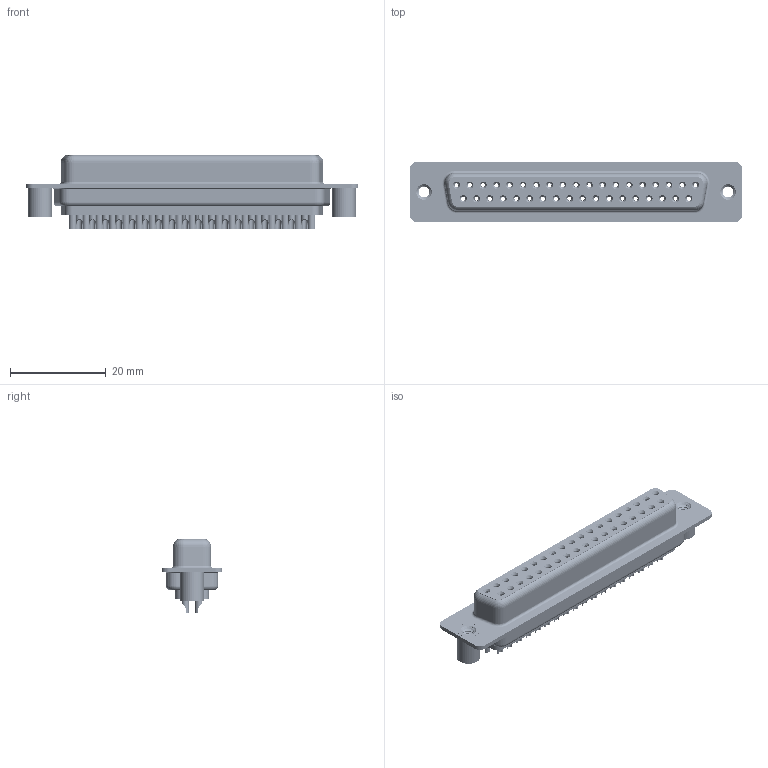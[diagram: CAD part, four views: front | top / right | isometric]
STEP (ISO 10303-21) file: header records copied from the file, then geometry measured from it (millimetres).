
FILE_DESCRIPTION (( 'STEP AP203' ), '1' );
FILE_NAME ('628-037-322-249.STEP', '2020-07-14T19:12:02', ( '' ), ( '' ), 'SwSTEP 2.0', 'SolidWorks 2020', '' );
FILE_SCHEMA (( 'CONFIG_CONTROL_DESIGN' ));
Length unit declared in the file: millimetre
Products named in the file (7): 628 Contact Row 2_22L; 628 Contact Row 1_22L; 628 4-40 Threaded Standoff BS; 628 Shell Front_37 Contacts; 628-037-322-249; 628 Shell Rear_37 Contacts; 628 Housing_37 LP
Assembly tree (42 placements, depth 2):
  628-037-322-249
    628 Housing_37 LP
    628 Shell Front_37 Contacts
    628 Shell Rear_37 Contacts
    628 Contact Row 1_22L  x19
    628 Contact Row 2_22L  x18
    628 4-40 Threaded Standoff BS  x2
Bounding box: 69.3 x 12.6 x 15.35 mm (x, y, z)
Volume: 5487.7 mm3; surface area: 13204.8 mm2
Topology: 42 solids, 42 shells, 3594 faces, 9111 edges, 5723 vertices
Faces by surface type: cylinder 1082, plane 844, bspline 746, torus 723, cone 199
Entity records: 30728 total; most frequent: CARTESIAN_POINT 8135, DIRECTION 4679, ORIENTED_EDGE 4136, EDGE_CURVE 2068, AXIS2_PLACEMENT_3D 1970, VERTEX_POINT 1310, EDGE_LOOP 1098, CIRCLE 1078
